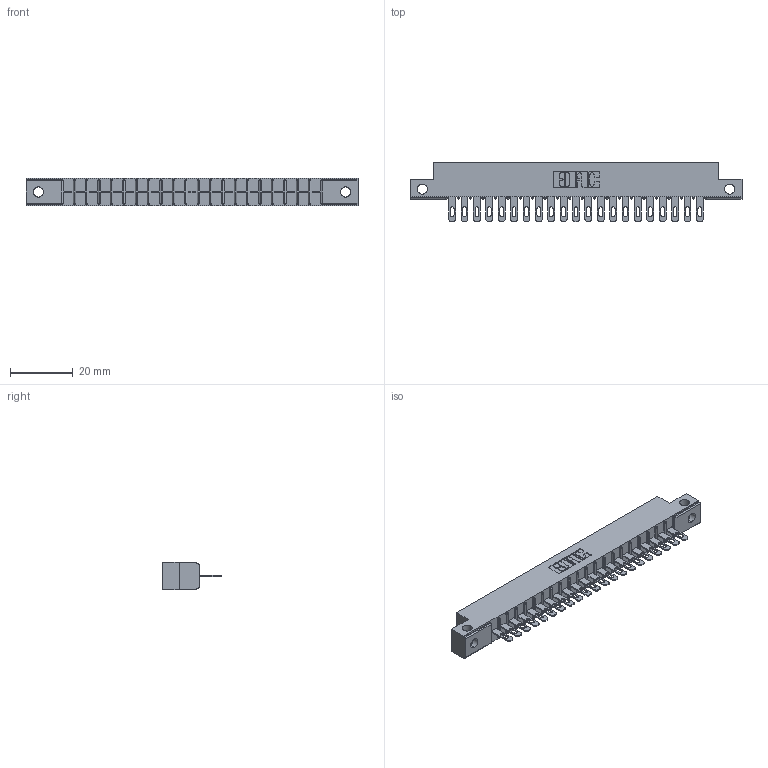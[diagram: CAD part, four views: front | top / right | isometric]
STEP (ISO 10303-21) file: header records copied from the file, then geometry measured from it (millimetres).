
FILE_DESCRIPTION (( 'STEP AP203' ), '1' );
FILE_NAME ('316-021-400-112.STEP', '2020-09-22T19:54:49', ( '' ), ( '' ), 'SwSTEP 2.0', 'SolidWorks 2020', '' );
FILE_SCHEMA (( 'CONFIG_CONTROL_DESIGN' ));
Length unit declared in the file: inch
Products named in the file (3): 306 Part_.128 Dia; 306-290-001_100; 316-021-400-112
Assembly tree (22 placements, depth 2):
  316-021-400-112
    306 Part_.128 Dia
    306-290-001_100  x21
Bounding box: 106.22 x 18.87 x 8.71 mm (x, y, z)
Volume: 7196.4 mm3; surface area: 10878.2 mm2
Topology: 22 solids, 22 shells, 1724 faces, 4867 edges, 3126 vertices
Faces by surface type: plane 1118, cylinder 522, sphere 84
Entity records: 22874 total; most frequent: CARTESIAN_POINT 3886, ORIENTED_EDGE 3806, DIRECTION 3773, EDGE_CURVE 1903, VECTOR 1459, LINE 1459, VERTEX_POINT 1206, AXIS2_PLACEMENT_3D 1157
